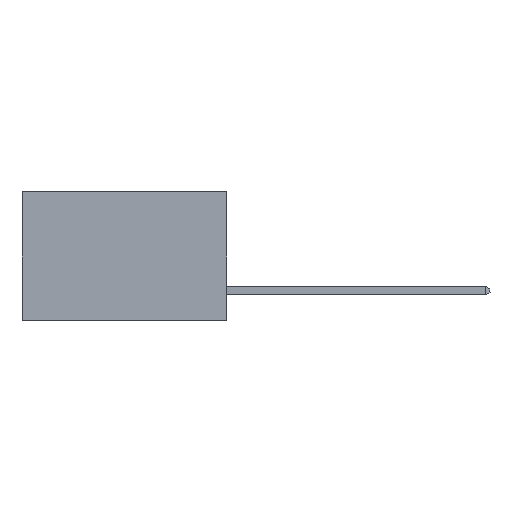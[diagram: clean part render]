
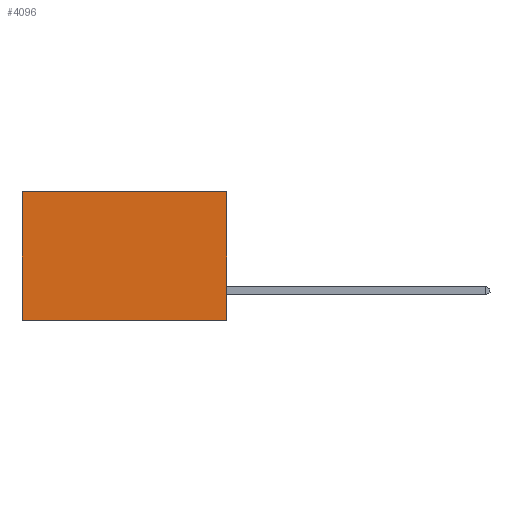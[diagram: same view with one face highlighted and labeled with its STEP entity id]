
A CAD part, left-side view. The second image highlights one B-rep face of the part: STEP entity #4096.
In plain terms, the highlighted planar face has unit normal (-1, 0, 0).
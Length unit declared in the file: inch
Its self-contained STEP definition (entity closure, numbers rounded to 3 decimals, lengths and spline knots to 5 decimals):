
#138 = DIRECTION ( 'NONE',  ( 0., 0., -1. ) ) ;
#226 = EDGE_LOOP ( 'NONE', ( #2242, #3896, #5185, #7246 ) ) ;
#444 = LINE ( 'NONE', #4710, #6007 ) ;
#1672 = VERTEX_POINT ( 'NONE', #8487 ) ;
#1827 = VECTOR ( 'NONE', #6587, 39.37008 ) ;
#2242 = ORIENTED_EDGE ( 'NONE', *, *, #2800, .T. ) ;
#2404 = VECTOR ( 'NONE', #7883, 39.37008 ) ;
#2800 = EDGE_CURVE ( 'NONE', #6775, #3394, #3274, .T. ) ;
#3274 = LINE ( 'NONE', #6662, #3486 ) ;
#3394 = VERTEX_POINT ( 'NONE', #8622 ) ;
#3486 = VECTOR ( 'NONE', #138, 39.37008 ) ;
#3534 = CARTESIAN_POINT ( 'NONE',  ( 0.277, 0.59, 0. ) ) ;
#3896 = ORIENTED_EDGE ( 'NONE', *, *, #5445, .F. ) ;
#4096 = ADVANCED_FACE ( 'NONE', ( #5802 ), #7072, .F. ) ;
#4354 = EDGE_CURVE ( 'NONE', #1672, #6775, #5688, .T. ) ;
#4559 = EDGE_CURVE ( 'NONE', #1672, #7656, #444, .T. ) ;
#4580 = DIRECTION ( 'NONE',  ( 0., 0., -1. ) ) ;
#4710 = CARTESIAN_POINT ( 'NONE',  ( 0.277, 0., -0.37 ) ) ;
#5185 = ORIENTED_EDGE ( 'NONE', *, *, #4559, .F. ) ;
#5364 = LINE ( 'NONE', #7267, #1827 ) ;
#5445 = EDGE_CURVE ( 'NONE', #7656, #3394, #5364, .T. ) ;
#5688 = LINE ( 'NONE', #7958, #2404 ) ;
#5802 = FACE_OUTER_BOUND ( 'NONE', #226, .T. ) ;
#6007 = VECTOR ( 'NONE', #4580, 39.37008 ) ;
#6587 = DIRECTION ( 'NONE',  ( 0., 1., 0. ) ) ;
#6662 = CARTESIAN_POINT ( 'NONE',  ( 0.277, 0.59, -0.37 ) ) ;
#6775 = VERTEX_POINT ( 'NONE', #3534 ) ;
#6790 = DIRECTION ( 'NONE',  ( 1., 0., 0. ) ) ;
#6929 = DIRECTION ( 'NONE',  ( 0., 0., -1. ) ) ;
#7072 = PLANE ( 'NONE',  #7382 ) ;
#7246 = ORIENTED_EDGE ( 'NONE', *, *, #4354, .T. ) ;
#7267 = CARTESIAN_POINT ( 'NONE',  ( 0.277, 0., -0.37 ) ) ;
#7382 = AXIS2_PLACEMENT_3D ( 'NONE', #7774, #6790, #6929 ) ;
#7656 = VERTEX_POINT ( 'NONE', #7918 ) ;
#7774 = CARTESIAN_POINT ( 'NONE',  ( 0.277, 0., -0.37 ) ) ;
#7883 = DIRECTION ( 'NONE',  ( 0., 1., 0. ) ) ;
#7918 = CARTESIAN_POINT ( 'NONE',  ( 0.277, 0., -0.37 ) ) ;
#7958 = CARTESIAN_POINT ( 'NONE',  ( 0.277, 0., 0. ) ) ;
#8487 = CARTESIAN_POINT ( 'NONE',  ( 0.277, 0., 0. ) ) ;
#8622 = CARTESIAN_POINT ( 'NONE',  ( 0.277, 0.59, -0.37 ) ) ;
